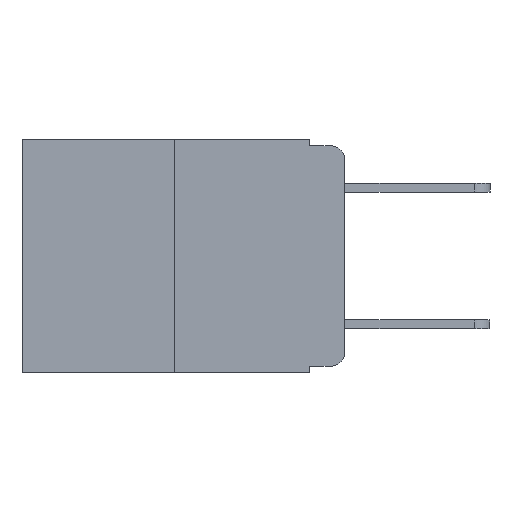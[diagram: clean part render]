
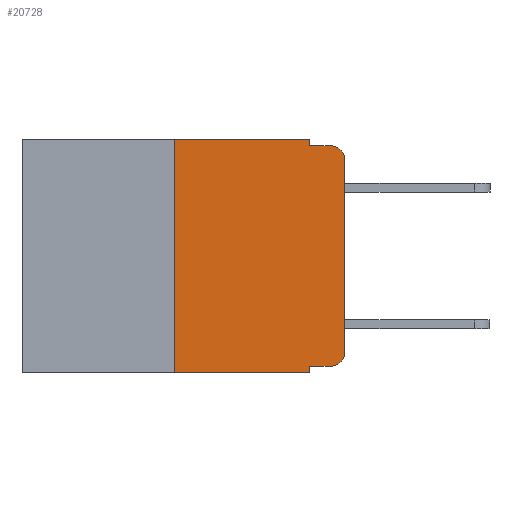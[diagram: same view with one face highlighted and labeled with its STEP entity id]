
A CAD part, left-side view. The second image highlights one B-rep face of the part: STEP entity #20728.
In plain terms, the highlighted planar face has unit normal (-1, 0, 0).
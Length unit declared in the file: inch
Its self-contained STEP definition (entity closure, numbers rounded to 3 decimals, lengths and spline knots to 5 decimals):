
#162 = VECTOR ( 'NONE', #13839, 39.37008 ) ;
#379 = VERTEX_POINT ( 'NONE', #10664 ) ;
#531 = CARTESIAN_POINT ( 'NONE',  ( 0., 0.02, -0.03 ) ) ;
#666 = VERTEX_POINT ( 'NONE', #1353 ) ;
#887 = LINE ( 'NONE', #7421, #162 ) ;
#1044 = ORIENTED_EDGE ( 'NONE', *, *, #19149, .F. ) ;
#1060 = VERTEX_POINT ( 'NONE', #11185 ) ;
#1071 = AXIS2_PLACEMENT_3D ( 'NONE', #14582, #6601, #17711 ) ;
#1353 = CARTESIAN_POINT ( 'NONE',  ( 0., 0.02, -0.01 ) ) ;
#1525 = DIRECTION ( 'NONE',  ( 0., 0., 1. ) ) ;
#1550 = DIRECTION ( 'NONE',  ( 0., -1., 0. ) ) ;
#2543 = EDGE_CURVE ( 'NONE', #19684, #17309, #20108, .T. ) ;
#2548 = DIRECTION ( 'NONE',  ( 0., 0., -1. ) ) ;
#2782 = LINE ( 'NONE', #20670, #6806 ) ;
#3075 = CARTESIAN_POINT ( 'NONE',  ( 0., 0.25, 0. ) ) ;
#3077 = VECTOR ( 'NONE', #4061, 39.37008 ) ;
#3720 = VERTEX_POINT ( 'NONE', #12238 ) ;
#3783 = EDGE_CURVE ( 'NONE', #17309, #666, #6245, .T. ) ;
#3954 = VERTEX_POINT ( 'NONE', #9873 ) ;
#4012 = VECTOR ( 'NONE', #1525, 39.37008 ) ;
#4061 = DIRECTION ( 'NONE',  ( 0., 0., 1. ) ) ;
#5215 = CARTESIAN_POINT ( 'NONE',  ( 0., 0.051, 0. ) ) ;
#5562 = AXIS2_PLACEMENT_3D ( 'NONE', #19766, #10449, #21223 ) ;
#5795 = ORIENTED_EDGE ( 'NONE', *, *, #3783, .T. ) ;
#6245 = CIRCLE ( 'NONE', #7590, 0.02 ) ;
#6385 = ORIENTED_EDGE ( 'NONE', *, *, #20035, .T. ) ;
#6601 = DIRECTION ( 'NONE',  ( 1., 0., 0. ) ) ;
#6604 = VECTOR ( 'NONE', #1550, 39.37008 ) ;
#6730 = CARTESIAN_POINT ( 'NONE',  ( 0., 0.25, 0. ) ) ;
#6734 = VERTEX_POINT ( 'NONE', #10434 ) ;
#6806 = VECTOR ( 'NONE', #17735, 39.37008 ) ;
#6827 = LINE ( 'NONE', #10322, #10626 ) ;
#7421 = CARTESIAN_POINT ( 'NONE',  ( 0., 0.051, 0. ) ) ;
#7558 = VECTOR ( 'NONE', #18587, 39.37008 ) ;
#7590 = AXIS2_PLACEMENT_3D ( 'NONE', #531, #12437, #2548 ) ;
#7694 = EDGE_CURVE ( 'NONE', #1060, #19684, #21059, .T. ) ;
#7856 = ORIENTED_EDGE ( 'NONE', *, *, #7694, .T. ) ;
#8402 = LINE ( 'NONE', #6730, #4012 ) ;
#8415 = EDGE_CURVE ( 'NONE', #3954, #1060, #15097, .T. ) ;
#8889 = VERTEX_POINT ( 'NONE', #12756 ) ;
#9651 = LINE ( 'NONE', #5215, #14370 ) ;
#9873 = CARTESIAN_POINT ( 'NONE',  ( 0., 0.051, -0.333 ) ) ;
#10148 = EDGE_CURVE ( 'NONE', #10740, #379, #6827, .T. ) ;
#10174 = EDGE_LOOP ( 'NONE', ( #12343, #5795, #17516, #14401, #13807, #1044, #6385, #12133, #12837, #7856 ) ) ;
#10322 = CARTESIAN_POINT ( 'NONE',  ( 0., 0.473, 0. ) ) ;
#10434 = CARTESIAN_POINT ( 'NONE',  ( 0., 0.25, -0.343 ) ) ;
#10449 = DIRECTION ( 'NONE',  ( -1., 0., 0. ) ) ;
#10626 = VECTOR ( 'NONE', #15012, 39.37008 ) ;
#10664 = CARTESIAN_POINT ( 'NONE',  ( 0., 0.051, 0. ) ) ;
#10740 = VERTEX_POINT ( 'NONE', #3075 ) ;
#11185 = CARTESIAN_POINT ( 'NONE',  ( 0., 0.02, -0.333 ) ) ;
#11464 = CARTESIAN_POINT ( 'NONE',  ( 0., 0., -0.313 ) ) ;
#12133 = ORIENTED_EDGE ( 'NONE', *, *, #12438, .F. ) ;
#12238 = CARTESIAN_POINT ( 'NONE',  ( 0., 0.051, -0.01 ) ) ;
#12343 = ORIENTED_EDGE ( 'NONE', *, *, #2543, .T. ) ;
#12437 = DIRECTION ( 'NONE',  ( -1., 0., 0. ) ) ;
#12438 = EDGE_CURVE ( 'NONE', #3954, #8889, #887, .T. ) ;
#12756 = CARTESIAN_POINT ( 'NONE',  ( 0., 0.051, -0.343 ) ) ;
#12791 = FACE_OUTER_BOUND ( 'NONE', #10174, .T. ) ;
#12837 = ORIENTED_EDGE ( 'NONE', *, *, #8415, .T. ) ;
#12965 = PLANE ( 'NONE',  #1071 ) ;
#13542 = CARTESIAN_POINT ( 'NONE',  ( 0., 0., 0. ) ) ;
#13807 = ORIENTED_EDGE ( 'NONE', *, *, #10148, .F. ) ;
#13839 = DIRECTION ( 'NONE',  ( 0., 0., -1. ) ) ;
#13892 = CARTESIAN_POINT ( 'NONE',  ( 0., 0.473, -0.343 ) ) ;
#14370 = VECTOR ( 'NONE', #14860, 39.37008 ) ;
#14401 = ORIENTED_EDGE ( 'NONE', *, *, #19262, .F. ) ;
#14582 = CARTESIAN_POINT ( 'NONE',  ( 0., 0.473, 0. ) ) ;
#14860 = DIRECTION ( 'NONE',  ( 0., 0., -1. ) ) ;
#14928 = CARTESIAN_POINT ( 'NONE',  ( 0., 0., -0.03 ) ) ;
#15012 = DIRECTION ( 'NONE',  ( 0., -1., 0. ) ) ;
#15097 = LINE ( 'NONE', #20850, #6604 ) ;
#16005 = LINE ( 'NONE', #13892, #7558 ) ;
#17309 = VERTEX_POINT ( 'NONE', #14928 ) ;
#17516 = ORIENTED_EDGE ( 'NONE', *, *, #20254, .F. ) ;
#17711 = DIRECTION ( 'NONE',  ( 0., 0., -1. ) ) ;
#17735 = DIRECTION ( 'NONE',  ( 0., -1., 0. ) ) ;
#18587 = DIRECTION ( 'NONE',  ( 0., -1., 0. ) ) ;
#19149 = EDGE_CURVE ( 'NONE', #6734, #10740, #8402, .T. ) ;
#19262 = EDGE_CURVE ( 'NONE', #379, #3720, #9651, .T. ) ;
#19684 = VERTEX_POINT ( 'NONE', #11464 ) ;
#19766 = CARTESIAN_POINT ( 'NONE',  ( 0., 0.02, -0.313 ) ) ;
#20035 = EDGE_CURVE ( 'NONE', #6734, #8889, #16005, .T. ) ;
#20108 = LINE ( 'NONE', #13542, #3077 ) ;
#20254 = EDGE_CURVE ( 'NONE', #3720, #666, #2782, .T. ) ;
#20670 = CARTESIAN_POINT ( 'NONE',  ( 0., 0.051, -0.01 ) ) ;
#20728 = ADVANCED_FACE ( 'NONE', ( #12791 ), #12965, .F. ) ;
#20850 = CARTESIAN_POINT ( 'NONE',  ( 0., 0.051, -0.333 ) ) ;
#21059 = CIRCLE ( 'NONE', #5562, 0.02 ) ;
#21223 = DIRECTION ( 'NONE',  ( 0., 0., -1. ) ) ;
